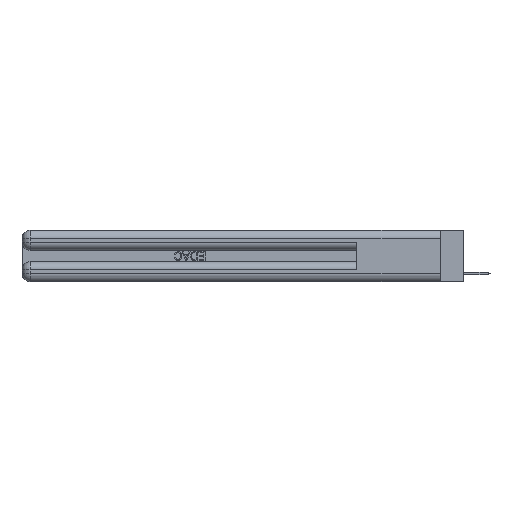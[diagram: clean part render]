
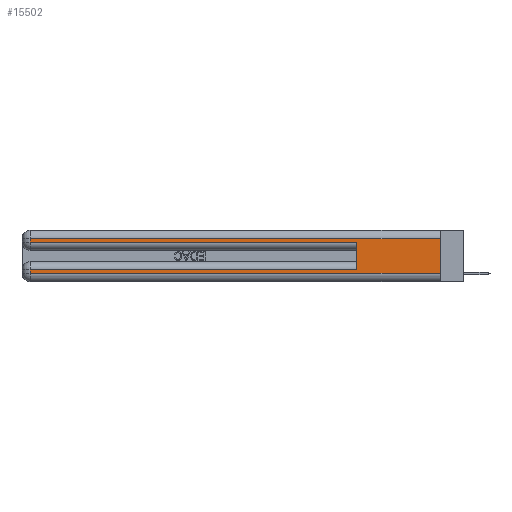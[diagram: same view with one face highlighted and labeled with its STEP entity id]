
A CAD part, left-side view. The second image highlights one B-rep face of the part: STEP entity #15502.
In plain terms, the highlighted planar face has unit normal (-1, 0, 0).
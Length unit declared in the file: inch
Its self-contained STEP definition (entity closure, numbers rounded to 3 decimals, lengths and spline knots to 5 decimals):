
#679 = FACE_OUTER_BOUND ( 'NONE', #12115, .T. ) ;
#1121 = CARTESIAN_POINT ( 'NONE',  ( 0., 0., 0.31 ) ) ;
#1211 = CARTESIAN_POINT ( 'NONE',  ( 0., 0., 0.37 ) ) ;
#1418 = DIRECTION ( 'NONE',  ( 0., -1., 0. ) ) ;
#1722 = ORIENTED_EDGE ( 'NONE', *, *, #7449, .F. ) ;
#2032 = VERTEX_POINT ( 'NONE', #4077 ) ;
#2115 = DIRECTION ( 'NONE',  ( 0., 0., -1. ) ) ;
#3186 = DIRECTION ( 'NONE',  ( 0., -1., 0. ) ) ;
#3981 = CARTESIAN_POINT ( 'NONE',  ( 0., 0.6, 0.145 ) ) ;
#3986 = LINE ( 'NONE', #22656, #10139 ) ;
#4077 = CARTESIAN_POINT ( 'NONE',  ( 0., 0.6, 0.085 ) ) ;
#4341 = CARTESIAN_POINT ( 'NONE',  ( 0., 0., 0.06 ) ) ;
#4454 = VERTEX_POINT ( 'NONE', #22598 ) ;
#4499 = CARTESIAN_POINT ( 'NONE',  ( 0., 2.94, 0.37 ) ) ;
#5270 = ORIENTED_EDGE ( 'NONE', *, *, #26279, .T. ) ;
#5373 = ORIENTED_EDGE ( 'NONE', *, *, #24211, .F. ) ;
#5868 = EDGE_CURVE ( 'NONE', #26881, #21974, #24984, .T. ) ;
#6167 = DIRECTION ( 'NONE',  ( 0., 1., 0. ) ) ;
#6761 = EDGE_CURVE ( 'NONE', #4454, #26881, #21830, .T. ) ;
#7010 = AXIS2_PLACEMENT_3D ( 'NONE', #27690, #10416, #12893 ) ;
#7449 = EDGE_CURVE ( 'NONE', #2032, #25159, #25280, .T. ) ;
#7555 = VERTEX_POINT ( 'NONE', #4341 ) ;
#8941 = LINE ( 'NONE', #28540, #9301 ) ;
#8942 = DIRECTION ( 'NONE',  ( 0., 0., 1. ) ) ;
#9301 = VECTOR ( 'NONE', #1418, 39.37008 ) ;
#10139 = VECTOR ( 'NONE', #6167, 39.37008 ) ;
#10235 = LINE ( 'NONE', #1211, #24164 ) ;
#10413 = CARTESIAN_POINT ( 'NONE',  ( 0., 0., 0.285 ) ) ;
#10416 = DIRECTION ( 'NONE',  ( 1., 0., 0. ) ) ;
#11137 = ORIENTED_EDGE ( 'NONE', *, *, #26024, .T. ) ;
#12115 = EDGE_LOOP ( 'NONE', ( #5373, #14974, #30980, #5270, #1722, #26338, #11137, #27644 ) ) ;
#12747 = DIRECTION ( 'NONE',  ( 0., 0., -1. ) ) ;
#12893 = DIRECTION ( 'NONE',  ( 0., 0., -1. ) ) ;
#13116 = CARTESIAN_POINT ( 'NONE',  ( 0., 2.94, 0.06 ) ) ;
#13322 = VECTOR ( 'NONE', #8942, 39.37008 ) ;
#14001 = LINE ( 'NONE', #10413, #20566 ) ;
#14974 = ORIENTED_EDGE ( 'NONE', *, *, #6761, .T. ) ;
#15502 = ADVANCED_FACE ( 'NONE', ( #679 ), #22700, .F. ) ;
#17496 = VERTEX_POINT ( 'NONE', #13116 ) ;
#19106 = EDGE_CURVE ( 'NONE', #2032, #19503, #3986, .T. ) ;
#19503 = VERTEX_POINT ( 'NONE', #21181 ) ;
#20083 = EDGE_CURVE ( 'NONE', #17496, #7555, #8941, .T. ) ;
#20301 = VECTOR ( 'NONE', #21067, 39.37008 ) ;
#20566 = VECTOR ( 'NONE', #3186, 39.37008 ) ;
#21067 = DIRECTION ( 'NONE',  ( 0., 1., 0. ) ) ;
#21181 = CARTESIAN_POINT ( 'NONE',  ( 0., 2.94, 0.085 ) ) ;
#21715 = VECTOR ( 'NONE', #2115, 39.37008 ) ;
#21830 = LINE ( 'NONE', #1121, #20301 ) ;
#21974 = VERTEX_POINT ( 'NONE', #25857 ) ;
#22598 = CARTESIAN_POINT ( 'NONE',  ( 0., 0., 0.31 ) ) ;
#22656 = CARTESIAN_POINT ( 'NONE',  ( 0., 0., 0.085 ) ) ;
#22700 = PLANE ( 'NONE',  #7010 ) ;
#24164 = VECTOR ( 'NONE', #31129, 39.37008 ) ;
#24211 = EDGE_CURVE ( 'NONE', #4454, #7555, #10235, .T. ) ;
#24570 = CARTESIAN_POINT ( 'NONE',  ( 0., 0.6, 0.285 ) ) ;
#24635 = VECTOR ( 'NONE', #12747, 39.37008 ) ;
#24984 = LINE ( 'NONE', #27551, #24635 ) ;
#25159 = VERTEX_POINT ( 'NONE', #24570 ) ;
#25280 = LINE ( 'NONE', #3981, #13322 ) ;
#25857 = CARTESIAN_POINT ( 'NONE',  ( 0., 2.94, 0.285 ) ) ;
#26024 = EDGE_CURVE ( 'NONE', #19503, #17496, #30679, .T. ) ;
#26279 = EDGE_CURVE ( 'NONE', #21974, #25159, #14001, .T. ) ;
#26338 = ORIENTED_EDGE ( 'NONE', *, *, #19106, .T. ) ;
#26881 = VERTEX_POINT ( 'NONE', #27603 ) ;
#27551 = CARTESIAN_POINT ( 'NONE',  ( 0., 2.94, 0.37 ) ) ;
#27603 = CARTESIAN_POINT ( 'NONE',  ( 0., 2.94, 0.31 ) ) ;
#27644 = ORIENTED_EDGE ( 'NONE', *, *, #20083, .T. ) ;
#27690 = CARTESIAN_POINT ( 'NONE',  ( 0., 0., 0.37 ) ) ;
#28540 = CARTESIAN_POINT ( 'NONE',  ( 0., 0., 0.06 ) ) ;
#30679 = LINE ( 'NONE', #4499, #21715 ) ;
#30980 = ORIENTED_EDGE ( 'NONE', *, *, #5868, .T. ) ;
#31129 = DIRECTION ( 'NONE',  ( 0., 0., -1. ) ) ;
